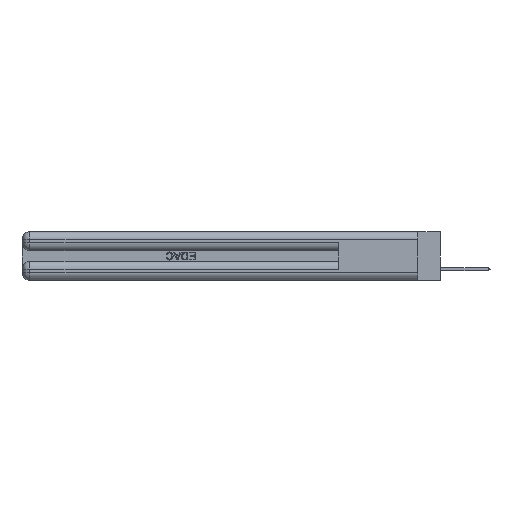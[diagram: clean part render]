
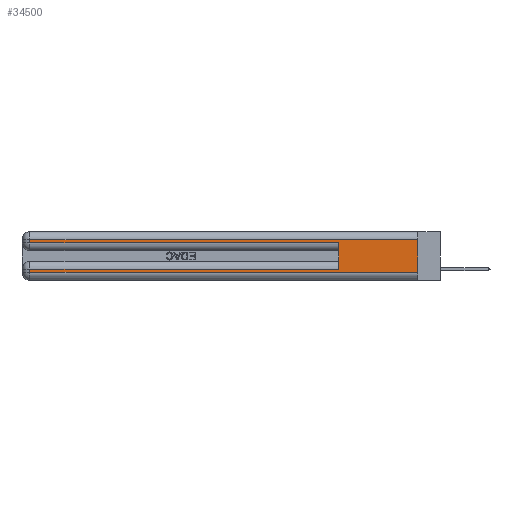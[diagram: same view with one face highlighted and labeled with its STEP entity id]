
A CAD part, left-side view. The second image highlights one B-rep face of the part: STEP entity #34500.
In plain terms, the highlighted planar face has unit normal (-1, 0, 0).
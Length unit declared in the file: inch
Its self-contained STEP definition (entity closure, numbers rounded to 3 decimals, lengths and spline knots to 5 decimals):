
#870 = EDGE_CURVE ( 'NONE', #24113, #23399, #36996, .T. ) ;
#1252 = LINE ( 'NONE', #34147, #14761 ) ;
#2357 = VECTOR ( 'NONE', #42830, 39.37008 ) ;
#2653 = ORIENTED_EDGE ( 'NONE', *, *, #4356, .T. ) ;
#2708 = ORIENTED_EDGE ( 'NONE', *, *, #14201, .F. ) ;
#2759 = DIRECTION ( 'NONE',  ( 0., 0., -1. ) ) ;
#2954 = DIRECTION ( 'NONE',  ( 0., 0., -1. ) ) ;
#3706 = VERTEX_POINT ( 'NONE', #41402 ) ;
#3774 = DIRECTION ( 'NONE',  ( 0., 0., -1. ) ) ;
#4356 = EDGE_CURVE ( 'NONE', #39775, #24323, #24092, .T. ) ;
#4358 = CARTESIAN_POINT ( 'NONE',  ( 0., 2.94, 0.37 ) ) ;
#5410 = DIRECTION ( 'NONE',  ( 1., 0., 0. ) ) ;
#5936 = VECTOR ( 'NONE', #37342, 39.37008 ) ;
#7924 = VECTOR ( 'NONE', #3774, 39.37008 ) ;
#10042 = ORIENTED_EDGE ( 'NONE', *, *, #11374, .T. ) ;
#11374 = EDGE_CURVE ( 'NONE', #41372, #3706, #1252, .T. ) ;
#12480 = VECTOR ( 'NONE', #2954, 39.37008 ) ;
#12559 = VECTOR ( 'NONE', #16302, 39.37008 ) ;
#12566 = EDGE_LOOP ( 'NONE', ( #19727, #41955, #38298, #10042, #2708, #31571, #20464, #2653 ) ) ;
#12810 = CARTESIAN_POINT ( 'NONE',  ( 0., 0.6, 0.145 ) ) ;
#14201 = EDGE_CURVE ( 'NONE', #17260, #3706, #38266, .T. ) ;
#14761 = VECTOR ( 'NONE', #27880, 39.37008 ) ;
#15470 = CARTESIAN_POINT ( 'NONE',  ( 0., 2.94, 0.31 ) ) ;
#15735 = VECTOR ( 'NONE', #31563, 39.37008 ) ;
#16302 = DIRECTION ( 'NONE',  ( 0., 1., 0. ) ) ;
#16406 = CARTESIAN_POINT ( 'NONE',  ( 0., 0., 0.31 ) ) ;
#17260 = VERTEX_POINT ( 'NONE', #21222 ) ;
#17350 = CARTESIAN_POINT ( 'NONE',  ( 0., 2.94, 0.285 ) ) ;
#17496 = CARTESIAN_POINT ( 'NONE',  ( 0., 2.94, 0.085 ) ) ;
#18012 = CARTESIAN_POINT ( 'NONE',  ( 0., 0., 0.37 ) ) ;
#18659 = AXIS2_PLACEMENT_3D ( 'NONE', #18012, #5410, #39000 ) ;
#19598 = CARTESIAN_POINT ( 'NONE',  ( 0., 2.94, 0.37 ) ) ;
#19727 = ORIENTED_EDGE ( 'NONE', *, *, #35075, .F. ) ;
#20464 = ORIENTED_EDGE ( 'NONE', *, *, #34707, .T. ) ;
#21203 = PLANE ( 'NONE',  #18659 ) ;
#21222 = CARTESIAN_POINT ( 'NONE',  ( 0., 0.6, 0.085 ) ) ;
#21521 = CARTESIAN_POINT ( 'NONE',  ( 0., 0., 0.085 ) ) ;
#21894 = FACE_OUTER_BOUND ( 'NONE', #12566, .T. ) ;
#23188 = EDGE_CURVE ( 'NONE', #23399, #41372, #31283, .T. ) ;
#23399 = VERTEX_POINT ( 'NONE', #15470 ) ;
#24092 = LINE ( 'NONE', #37623, #5936 ) ;
#24113 = VERTEX_POINT ( 'NONE', #16406 ) ;
#24323 = VERTEX_POINT ( 'NONE', #26138 ) ;
#25871 = CARTESIAN_POINT ( 'NONE',  ( 0., 2.94, 0.06 ) ) ;
#26138 = CARTESIAN_POINT ( 'NONE',  ( 0., 0., 0.06 ) ) ;
#26183 = CARTESIAN_POINT ( 'NONE',  ( 0., 0., 0.37 ) ) ;
#26573 = LINE ( 'NONE', #19598, #33796 ) ;
#27667 = LINE ( 'NONE', #21521, #15735 ) ;
#27880 = DIRECTION ( 'NONE',  ( 0., -1., 0. ) ) ;
#31193 = VERTEX_POINT ( 'NONE', #17496 ) ;
#31283 = LINE ( 'NONE', #4358, #7924 ) ;
#31563 = DIRECTION ( 'NONE',  ( 0., 1., 0. ) ) ;
#31571 = ORIENTED_EDGE ( 'NONE', *, *, #42142, .T. ) ;
#33796 = VECTOR ( 'NONE', #2759, 39.37008 ) ;
#34147 = CARTESIAN_POINT ( 'NONE',  ( 0., 0., 0.285 ) ) ;
#34500 = ADVANCED_FACE ( 'NONE', ( #21894 ), #21203, .F. ) ;
#34707 = EDGE_CURVE ( 'NONE', #31193, #39775, #26573, .T. ) ;
#35075 = EDGE_CURVE ( 'NONE', #24113, #24323, #40623, .T. ) ;
#36996 = LINE ( 'NONE', #39339, #12559 ) ;
#37342 = DIRECTION ( 'NONE',  ( 0., -1., 0. ) ) ;
#37623 = CARTESIAN_POINT ( 'NONE',  ( 0., 0., 0.06 ) ) ;
#38266 = LINE ( 'NONE', #12810, #2357 ) ;
#38298 = ORIENTED_EDGE ( 'NONE', *, *, #23188, .T. ) ;
#39000 = DIRECTION ( 'NONE',  ( 0., 0., -1. ) ) ;
#39339 = CARTESIAN_POINT ( 'NONE',  ( 0., 0., 0.31 ) ) ;
#39775 = VERTEX_POINT ( 'NONE', #25871 ) ;
#40623 = LINE ( 'NONE', #26183, #12480 ) ;
#41372 = VERTEX_POINT ( 'NONE', #17350 ) ;
#41402 = CARTESIAN_POINT ( 'NONE',  ( 0., 0.6, 0.285 ) ) ;
#41955 = ORIENTED_EDGE ( 'NONE', *, *, #870, .T. ) ;
#42142 = EDGE_CURVE ( 'NONE', #17260, #31193, #27667, .T. ) ;
#42830 = DIRECTION ( 'NONE',  ( 0., 0., 1. ) ) ;
